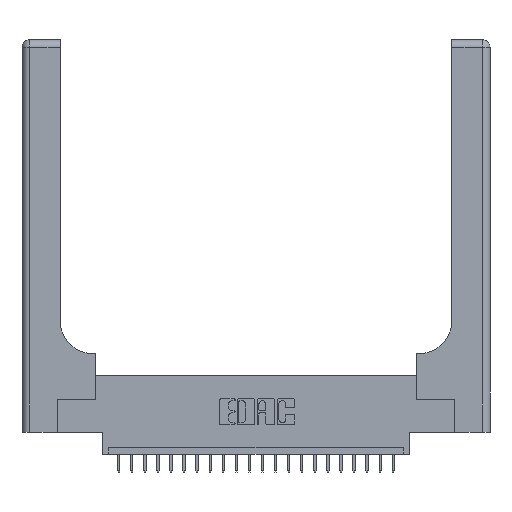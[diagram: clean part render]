
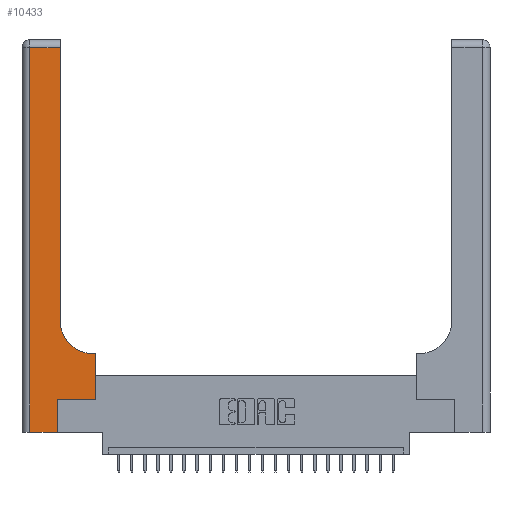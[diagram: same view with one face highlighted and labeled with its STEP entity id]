
A CAD part, top view. The second image highlights one B-rep face of the part: STEP entity #10433.
In plain terms, the highlighted planar face has unit normal (0, 0, 1).
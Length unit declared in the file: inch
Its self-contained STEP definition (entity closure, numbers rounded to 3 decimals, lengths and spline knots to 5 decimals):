
#504 = CARTESIAN_POINT ( 'NONE',  ( 0., 2.94, 0.37 ) ) ;
#1621 = VECTOR ( 'NONE', #14631, 39.37008 ) ;
#1670 = ORIENTED_EDGE ( 'NONE', *, *, #19702, .T. ) ;
#1749 = ORIENTED_EDGE ( 'NONE', *, *, #5189, .T. ) ;
#1880 = EDGE_CURVE ( 'NONE', #24413, #20477, #11889, .T. ) ;
#3171 = DIRECTION ( 'NONE',  ( 1., 0., 0. ) ) ;
#4882 = DIRECTION ( 'NONE',  ( -1., 0., 0. ) ) ;
#4991 = ORIENTED_EDGE ( 'NONE', *, *, #14118, .T. ) ;
#5024 = CARTESIAN_POINT ( 'NONE',  ( 0.5585, 0.25, 0.37 ) ) ;
#5189 = EDGE_CURVE ( 'NONE', #20477, #18530, #5338, .T. ) ;
#5338 = LINE ( 'NONE', #12750, #7470 ) ;
#5430 = CARTESIAN_POINT ( 'NONE',  ( 0.2915, 0.6, 0.37 ) ) ;
#5820 = EDGE_LOOP ( 'NONE', ( #1670, #8747, #24176, #8374, #5868, #1749, #4991, #16677, #24047 ) ) ;
#5868 = ORIENTED_EDGE ( 'NONE', *, *, #1880, .T. ) ;
#6199 = CARTESIAN_POINT ( 'NONE',  ( 0.269, 0., 0.37 ) ) ;
#7180 = VECTOR ( 'NONE', #15372, 39.37008 ) ;
#7462 = VERTEX_POINT ( 'NONE', #8828 ) ;
#7470 = VECTOR ( 'NONE', #3171, 39.37008 ) ;
#7762 = LINE ( 'NONE', #11821, #23502 ) ;
#8374 = ORIENTED_EDGE ( 'NONE', *, *, #11044, .T. ) ;
#8404 = CIRCLE ( 'NONE', #15106, 0.25 ) ;
#8612 = FACE_OUTER_BOUND ( 'NONE', #5820, .T. ) ;
#8747 = ORIENTED_EDGE ( 'NONE', *, *, #22322, .T. ) ;
#8828 = CARTESIAN_POINT ( 'NONE',  ( 0.06, 2.94, 0.37 ) ) ;
#9116 = CARTESIAN_POINT ( 'NONE',  ( 0.5585, 0.6, 0.37 ) ) ;
#9340 = DIRECTION ( 'NONE',  ( 1., 0., 0. ) ) ;
#9555 = CARTESIAN_POINT ( 'NONE',  ( 0.2915, 0.85, 0.37 ) ) ;
#10433 = ADVANCED_FACE ( 'NONE', ( #8612 ), #21920, .F. ) ;
#10618 = DIRECTION ( 'NONE',  ( 1., 0., 0. ) ) ;
#10706 = CARTESIAN_POINT ( 'NONE',  ( 0., 3., 0.37 ) ) ;
#10796 = EDGE_CURVE ( 'NONE', #14300, #20642, #11374, .T. ) ;
#10863 = CARTESIAN_POINT ( 'NONE',  ( 0., 0., 0.37 ) ) ;
#10956 = VERTEX_POINT ( 'NONE', #22200 ) ;
#10999 = CARTESIAN_POINT ( 'NONE',  ( 0.06, 0., 0.37 ) ) ;
#11044 = EDGE_CURVE ( 'NONE', #18025, #24413, #23949, .T. ) ;
#11127 = EDGE_CURVE ( 'NONE', #7462, #18025, #7762, .T. ) ;
#11280 = EDGE_CURVE ( 'NONE', #20642, #17017, #8404, .T. ) ;
#11374 = LINE ( 'NONE', #5430, #22288 ) ;
#11821 = CARTESIAN_POINT ( 'NONE',  ( 0.06, 3., 0.37 ) ) ;
#11889 = LINE ( 'NONE', #6199, #7180 ) ;
#12552 = CARTESIAN_POINT ( 'NONE',  ( 0.5585, 0.25, 0.37 ) ) ;
#12571 = DIRECTION ( 'NONE',  ( 0., 1., 0. ) ) ;
#12750 = CARTESIAN_POINT ( 'NONE',  ( 0.269, 0.25, 0.37 ) ) ;
#13473 = DIRECTION ( 'NONE',  ( -1., 0., 0. ) ) ;
#14118 = EDGE_CURVE ( 'NONE', #18530, #14300, #14432, .T. ) ;
#14300 = VERTEX_POINT ( 'NONE', #9116 ) ;
#14432 = LINE ( 'NONE', #5024, #18780 ) ;
#14631 = DIRECTION ( 'NONE',  ( 0., 1., 0. ) ) ;
#14965 = DIRECTION ( 'NONE',  ( -1., 0., 0. ) ) ;
#15025 = CARTESIAN_POINT ( 'NONE',  ( 0.5415, 0.85, 0.37 ) ) ;
#15106 = AXIS2_PLACEMENT_3D ( 'NONE', #15025, #19160, #9340 ) ;
#15372 = DIRECTION ( 'NONE',  ( 0., 1., 0. ) ) ;
#16168 = DIRECTION ( 'NONE',  ( 0., 0., -1. ) ) ;
#16677 = ORIENTED_EDGE ( 'NONE', *, *, #10796, .T. ) ;
#16879 = VECTOR ( 'NONE', #13473, 39.37008 ) ;
#17017 = VERTEX_POINT ( 'NONE', #9555 ) ;
#17438 = DIRECTION ( 'NONE',  ( 0., -1., 0. ) ) ;
#18006 = CARTESIAN_POINT ( 'NONE',  ( 0.5415, 0.6, 0.37 ) ) ;
#18025 = VERTEX_POINT ( 'NONE', #10999 ) ;
#18436 = CARTESIAN_POINT ( 'NONE',  ( 0.269, 0., 0.37 ) ) ;
#18530 = VERTEX_POINT ( 'NONE', #12552 ) ;
#18780 = VECTOR ( 'NONE', #12571, 39.37008 ) ;
#19160 = DIRECTION ( 'NONE',  ( 0., 0., -1. ) ) ;
#19702 = EDGE_CURVE ( 'NONE', #17017, #10956, #20281, .T. ) ;
#20281 = LINE ( 'NONE', #24117, #1621 ) ;
#20339 = VECTOR ( 'NONE', #10618, 39.37008 ) ;
#20477 = VERTEX_POINT ( 'NONE', #21670 ) ;
#20642 = VERTEX_POINT ( 'NONE', #18006 ) ;
#21473 = LINE ( 'NONE', #504, #16879 ) ;
#21670 = CARTESIAN_POINT ( 'NONE',  ( 0.269, 0.25, 0.37 ) ) ;
#21920 = PLANE ( 'NONE',  #23897 ) ;
#22200 = CARTESIAN_POINT ( 'NONE',  ( 0.2915, 2.94, 0.37 ) ) ;
#22288 = VECTOR ( 'NONE', #14965, 39.37008 ) ;
#22322 = EDGE_CURVE ( 'NONE', #10956, #7462, #21473, .T. ) ;
#23502 = VECTOR ( 'NONE', #17438, 39.37008 ) ;
#23897 = AXIS2_PLACEMENT_3D ( 'NONE', #10706, #16168, #4882 ) ;
#23949 = LINE ( 'NONE', #10863, #20339 ) ;
#24047 = ORIENTED_EDGE ( 'NONE', *, *, #11280, .T. ) ;
#24117 = CARTESIAN_POINT ( 'NONE',  ( 0.2915, 3., 0.37 ) ) ;
#24176 = ORIENTED_EDGE ( 'NONE', *, *, #11127, .T. ) ;
#24413 = VERTEX_POINT ( 'NONE', #18436 ) ;
